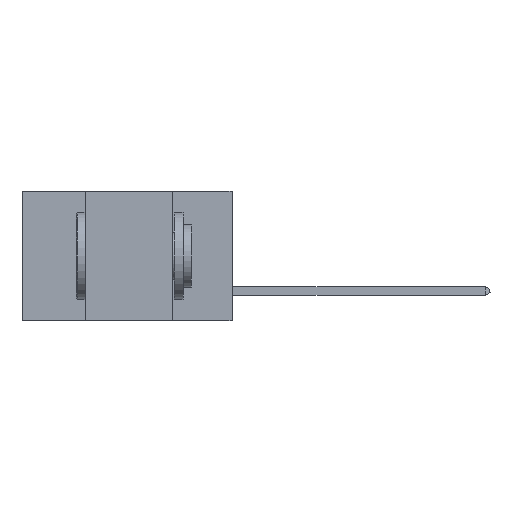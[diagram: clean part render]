
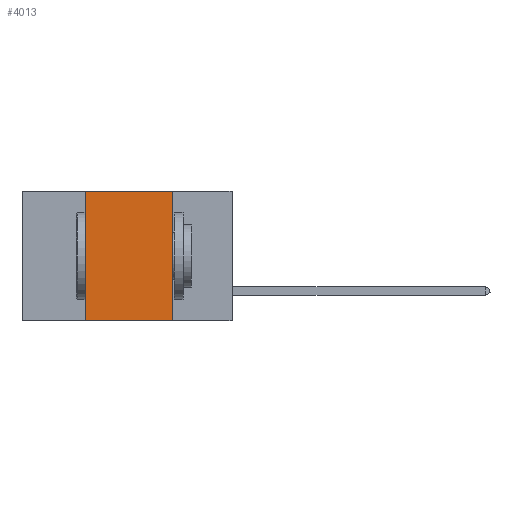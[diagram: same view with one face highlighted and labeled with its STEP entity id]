
A CAD part, left-side view. The second image highlights one B-rep face of the part: STEP entity #4013.
In plain terms, the highlighted planar face has unit normal (-1, 0, 0).
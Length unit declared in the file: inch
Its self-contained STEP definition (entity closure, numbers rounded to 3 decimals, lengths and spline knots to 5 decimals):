
#21 = ORIENTED_EDGE ( 'NONE', *, *, #494, .F. ) ;
#84 = DIRECTION ( 'NONE',  ( 0., 0., 1. ) ) ;
#232 = CARTESIAN_POINT ( 'NONE',  ( 0., 0.42, -0.37 ) ) ;
#494 = EDGE_CURVE ( 'NONE', #9932, #13913, #3744, .T. ) ;
#2508 = VECTOR ( 'NONE', #19351, 39.37008 ) ;
#2715 = VERTEX_POINT ( 'NONE', #232 ) ;
#2766 = PLANE ( 'NONE',  #17095 ) ;
#2901 = EDGE_CURVE ( 'NONE', #13913, #9039, #6337, .T. ) ;
#3744 = LINE ( 'NONE', #21255, #10784 ) ;
#4013 = ADVANCED_FACE ( 'NONE', ( #14409 ), #2766, .F. ) ;
#4145 = CARTESIAN_POINT ( 'NONE',  ( 0., 0.17, 0. ) ) ;
#5615 = CARTESIAN_POINT ( 'NONE',  ( 0., 0.17, -0.37 ) ) ;
#6337 = LINE ( 'NONE', #18258, #15817 ) ;
#6401 = EDGE_CURVE ( 'NONE', #2715, #9039, #7123, .T. ) ;
#7123 = LINE ( 'NONE', #10591, #2508 ) ;
#7542 = EDGE_CURVE ( 'NONE', #2715, #9932, #12765, .T. ) ;
#8696 = VECTOR ( 'NONE', #84, 39.37008 ) ;
#9039 = VERTEX_POINT ( 'NONE', #5615 ) ;
#9932 = VERTEX_POINT ( 'NONE', #22066 ) ;
#9967 = DIRECTION ( 'NONE',  ( 0., 0., -1. ) ) ;
#10591 = CARTESIAN_POINT ( 'NONE',  ( 0., 0.6, -0.37 ) ) ;
#10784 = VECTOR ( 'NONE', #17421, 39.37008 ) ;
#12765 = LINE ( 'NONE', #20953, #8696 ) ;
#13237 = DIRECTION ( 'NONE',  ( 1., 0., 0. ) ) ;
#13913 = VERTEX_POINT ( 'NONE', #4145 ) ;
#14409 = FACE_OUTER_BOUND ( 'NONE', #19706, .T. ) ;
#15436 = ORIENTED_EDGE ( 'NONE', *, *, #2901, .F. ) ;
#15817 = VECTOR ( 'NONE', #19769, 39.37008 ) ;
#17095 = AXIS2_PLACEMENT_3D ( 'NONE', #20366, #13237, #9967 ) ;
#17421 = DIRECTION ( 'NONE',  ( 0., -1., 0. ) ) ;
#18258 = CARTESIAN_POINT ( 'NONE',  ( 0., 0.17, 0. ) ) ;
#18357 = ORIENTED_EDGE ( 'NONE', *, *, #6401, .T. ) ;
#19351 = DIRECTION ( 'NONE',  ( 0., -1., 0. ) ) ;
#19666 = ORIENTED_EDGE ( 'NONE', *, *, #7542, .F. ) ;
#19706 = EDGE_LOOP ( 'NONE', ( #15436, #21, #19666, #18357 ) ) ;
#19769 = DIRECTION ( 'NONE',  ( 0., 0., -1. ) ) ;
#20366 = CARTESIAN_POINT ( 'NONE',  ( 0., 0.6, 0. ) ) ;
#20953 = CARTESIAN_POINT ( 'NONE',  ( 0., 0.42, 0. ) ) ;
#21255 = CARTESIAN_POINT ( 'NONE',  ( 0., 0.6, 0. ) ) ;
#22066 = CARTESIAN_POINT ( 'NONE',  ( 0., 0.42, 0. ) ) ;
